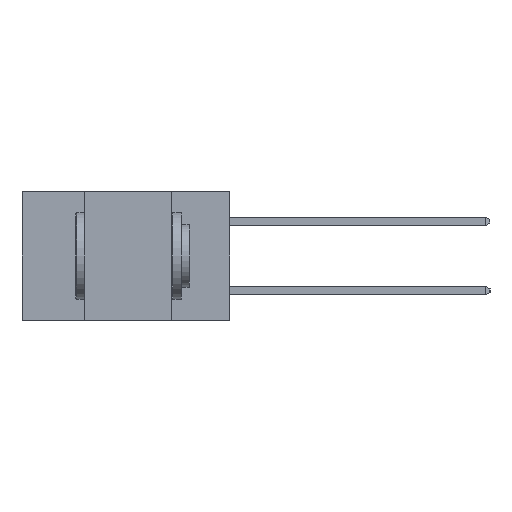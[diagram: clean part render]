
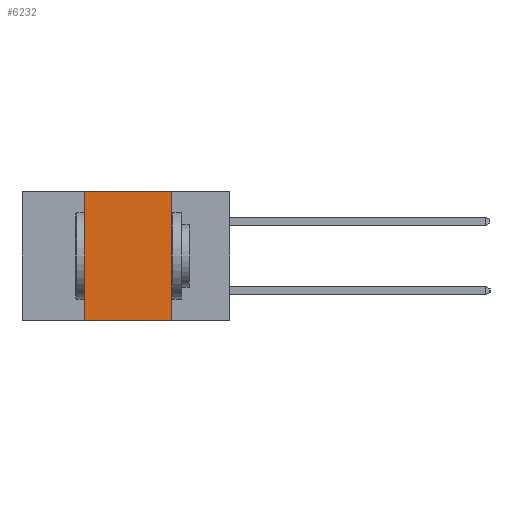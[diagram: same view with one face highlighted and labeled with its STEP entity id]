
A CAD part, left-side view. The second image highlights one B-rep face of the part: STEP entity #6232.
In plain terms, the highlighted planar face has unit normal (-1, 0, 0).
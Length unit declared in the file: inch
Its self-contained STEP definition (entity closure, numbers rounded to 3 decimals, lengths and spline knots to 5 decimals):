
#699 = VECTOR ( 'NONE', #2277, 39.37008 ) ;
#1154 = LINE ( 'NONE', #12541, #14416 ) ;
#1184 = VERTEX_POINT ( 'NONE', #9973 ) ;
#1471 = EDGE_CURVE ( 'NONE', #10422, #1184, #1154, .T. ) ;
#1509 = LINE ( 'NONE', #13734, #11794 ) ;
#1940 = VERTEX_POINT ( 'NONE', #7556 ) ;
#2157 = ORIENTED_EDGE ( 'NONE', *, *, #15479, .T. ) ;
#2277 = DIRECTION ( 'NONE',  ( 0., -1., 0. ) ) ;
#2370 = EDGE_CURVE ( 'NONE', #1184, #8566, #4221, .T. ) ;
#3087 = ORIENTED_EDGE ( 'NONE', *, *, #3243, .F. ) ;
#3243 = EDGE_CURVE ( 'NONE', #8566, #1940, #1509, .T. ) ;
#3499 = CARTESIAN_POINT ( 'NONE',  ( 0., 0.17, 0. ) ) ;
#3541 = EDGE_LOOP ( 'NONE', ( #3087, #11132, #12827, #2157 ) ) ;
#3805 = CARTESIAN_POINT ( 'NONE',  ( 0., 0.6, 0. ) ) ;
#4221 = LINE ( 'NONE', #3805, #699 ) ;
#6232 = ADVANCED_FACE ( 'NONE', ( #7507 ), #12927, .F. ) ;
#6503 = DIRECTION ( 'NONE',  ( 0., 0., 1. ) ) ;
#7507 = FACE_OUTER_BOUND ( 'NONE', #3541, .T. ) ;
#7556 = CARTESIAN_POINT ( 'NONE',  ( 0., 0.17, -0.37 ) ) ;
#7932 = CARTESIAN_POINT ( 'NONE',  ( 0., 0.6, -0.37 ) ) ;
#8271 = CARTESIAN_POINT ( 'NONE',  ( 0., 0.42, -0.37 ) ) ;
#8566 = VERTEX_POINT ( 'NONE', #3499 ) ;
#9000 = VECTOR ( 'NONE', #10483, 39.37008 ) ;
#9856 = AXIS2_PLACEMENT_3D ( 'NONE', #12888, #12793, #12684 ) ;
#9973 = CARTESIAN_POINT ( 'NONE',  ( 0., 0.42, 0. ) ) ;
#10422 = VERTEX_POINT ( 'NONE', #8271 ) ;
#10483 = DIRECTION ( 'NONE',  ( 0., -1., 0. ) ) ;
#11132 = ORIENTED_EDGE ( 'NONE', *, *, #2370, .F. ) ;
#11794 = VECTOR ( 'NONE', #12948, 39.37008 ) ;
#12407 = LINE ( 'NONE', #7932, #9000 ) ;
#12541 = CARTESIAN_POINT ( 'NONE',  ( 0., 0.42, -0.37 ) ) ;
#12684 = DIRECTION ( 'NONE',  ( 0., 0., -1. ) ) ;
#12793 = DIRECTION ( 'NONE',  ( 1., 0., 0. ) ) ;
#12827 = ORIENTED_EDGE ( 'NONE', *, *, #1471, .F. ) ;
#12888 = CARTESIAN_POINT ( 'NONE',  ( 0., 0.6, 0. ) ) ;
#12927 = PLANE ( 'NONE',  #9856 ) ;
#12948 = DIRECTION ( 'NONE',  ( 0., 0., -1. ) ) ;
#13734 = CARTESIAN_POINT ( 'NONE',  ( 0., 0.17, -0.37 ) ) ;
#14416 = VECTOR ( 'NONE', #6503, 39.37008 ) ;
#15479 = EDGE_CURVE ( 'NONE', #10422, #1940, #12407, .T. ) ;
